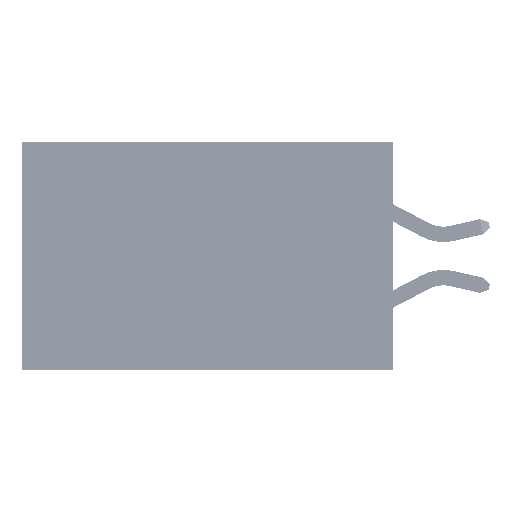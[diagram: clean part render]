
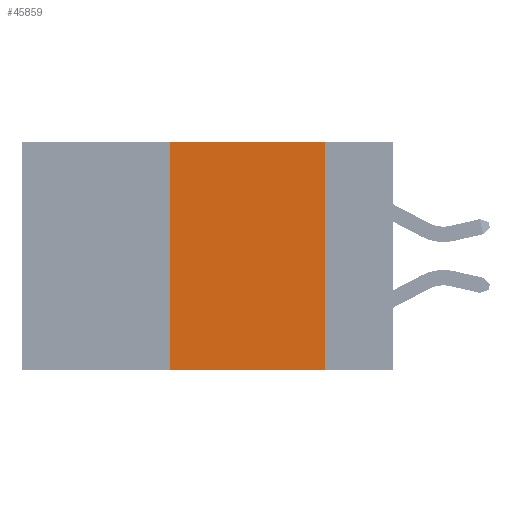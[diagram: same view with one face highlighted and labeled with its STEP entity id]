
A CAD part, left-side view. The second image highlights one B-rep face of the part: STEP entity #45859.
In plain terms, the highlighted planar face has unit normal (-1, 0, 0).
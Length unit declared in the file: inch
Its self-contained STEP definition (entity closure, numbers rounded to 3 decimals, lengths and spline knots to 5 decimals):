
#1007 = VERTEX_POINT ( 'NONE', #4753 ) ;
#1538 = CARTESIAN_POINT ( 'NONE',  ( 0., 0.36, -0.37 ) ) ;
#4648 = DIRECTION ( 'NONE',  ( 0., 0., -1. ) ) ;
#4753 = CARTESIAN_POINT ( 'NONE',  ( 0., 0.11, 0. ) ) ;
#8150 = EDGE_CURVE ( 'NONE', #25288, #34919, #34914, .T. ) ;
#9816 = LINE ( 'NONE', #26750, #39666 ) ;
#13734 = ORIENTED_EDGE ( 'NONE', *, *, #15116, .F. ) ;
#15116 = EDGE_CURVE ( 'NONE', #1007, #34919, #36285, .T. ) ;
#15562 = DIRECTION ( 'NONE',  ( 1., 0., 0. ) ) ;
#16625 = AXIS2_PLACEMENT_3D ( 'NONE', #45036, #15562, #19250 ) ;
#19119 = CARTESIAN_POINT ( 'NONE',  ( 0., 0.36, 0. ) ) ;
#19250 = DIRECTION ( 'NONE',  ( 0., 0., -1. ) ) ;
#20005 = CARTESIAN_POINT ( 'NONE',  ( 0., 0.6, -0.37 ) ) ;
#20311 = CARTESIAN_POINT ( 'NONE',  ( 0., 0.6, 0. ) ) ;
#21381 = VECTOR ( 'NONE', #4648, 39.37008 ) ;
#22996 = EDGE_CURVE ( 'NONE', #27889, #1007, #24381, .T. ) ;
#23131 = ORIENTED_EDGE ( 'NONE', *, *, #40542, .F. ) ;
#23387 = DIRECTION ( 'NONE',  ( 0., 0., 1. ) ) ;
#24381 = LINE ( 'NONE', #20311, #25518 ) ;
#25288 = VERTEX_POINT ( 'NONE', #1538 ) ;
#25518 = VECTOR ( 'NONE', #27694, 39.37008 ) ;
#25675 = EDGE_LOOP ( 'NONE', ( #13734, #32552, #23131, #45260 ) ) ;
#26750 = CARTESIAN_POINT ( 'NONE',  ( 0., 0.36, 0. ) ) ;
#27451 = VECTOR ( 'NONE', #31500, 39.37008 ) ;
#27694 = DIRECTION ( 'NONE',  ( 0., -1., 0. ) ) ;
#27889 = VERTEX_POINT ( 'NONE', #19119 ) ;
#28421 = CARTESIAN_POINT ( 'NONE',  ( 0., 0.11, -0.37 ) ) ;
#30038 = CARTESIAN_POINT ( 'NONE',  ( 0., 0.11, 0. ) ) ;
#31500 = DIRECTION ( 'NONE',  ( 0., -1., 0. ) ) ;
#32423 = FACE_OUTER_BOUND ( 'NONE', #25675, .T. ) ;
#32552 = ORIENTED_EDGE ( 'NONE', *, *, #22996, .F. ) ;
#34914 = LINE ( 'NONE', #20005, #27451 ) ;
#34919 = VERTEX_POINT ( 'NONE', #28421 ) ;
#36285 = LINE ( 'NONE', #30038, #21381 ) ;
#37529 = PLANE ( 'NONE',  #16625 ) ;
#39666 = VECTOR ( 'NONE', #23387, 39.37008 ) ;
#40542 = EDGE_CURVE ( 'NONE', #25288, #27889, #9816, .T. ) ;
#45036 = CARTESIAN_POINT ( 'NONE',  ( 0., 0.6, 0. ) ) ;
#45260 = ORIENTED_EDGE ( 'NONE', *, *, #8150, .T. ) ;
#45859 = ADVANCED_FACE ( 'NONE', ( #32423 ), #37529, .F. ) ;
